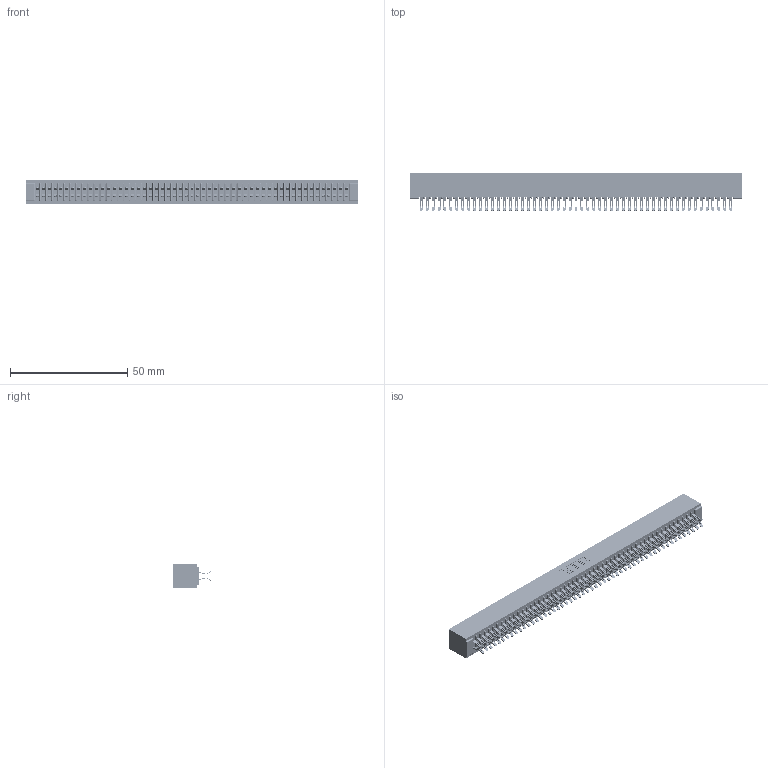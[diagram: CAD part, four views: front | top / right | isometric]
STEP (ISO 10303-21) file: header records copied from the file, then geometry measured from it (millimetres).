
FILE_DESCRIPTION (( 'STEP AP203' ), '1' );
FILE_NAME ('391-106-555-201.STEP', '2018-08-09T20:52:28', ( '' ), ( '' ), 'SwSTEP 2.0', 'SolidWorks 2016', '' );
FILE_SCHEMA (( 'CONFIG_CONTROL_DESIGN' ));
Length unit declared in the file: inch
Products named in the file (3): 341 Part_No Mounting Lugs; 341-292-001_341-292-155; 391-106-555-201
Assembly tree (107 placements, depth 2):
  391-106-555-201
    341 Part_No Mounting Lugs
    341-292-001_341-292-155  x106
Bounding box: 141.6 x 16.31 x 10.16 mm (x, y, z)
Volume: 10837.1 mm3; surface area: 21111.8 mm2
Topology: 107 solids, 107 shells, 8376 faces, 25043 edges, 16302 vertices
Faces by surface type: plane 4516, cylinder 3648, sphere 108, torus 104
Entity records: 62868 total; most frequent: CARTESIAN_POINT 10465, ORIENTED_EDGE 10390, DIRECTION 10137, EDGE_CURVE 5195, LINE 4197, VECTOR 4197, VERTEX_POINT 3282, AXIS2_PLACEMENT_3D 2970
